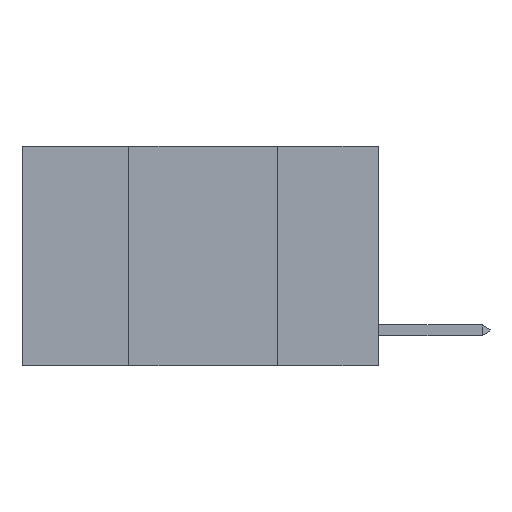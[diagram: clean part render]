
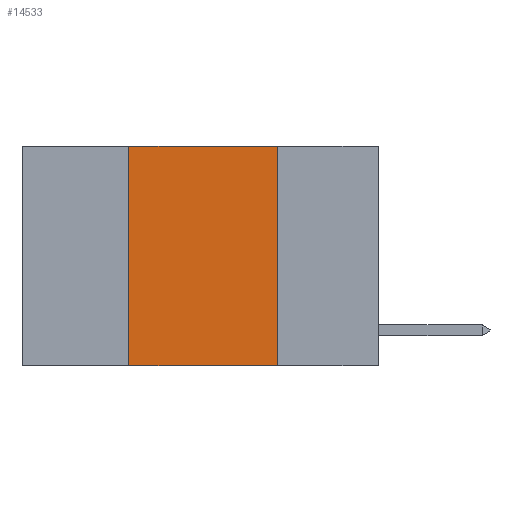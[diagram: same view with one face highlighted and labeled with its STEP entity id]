
A CAD part, left-side view. The second image highlights one B-rep face of the part: STEP entity #14533.
In plain terms, the highlighted planar face has unit normal (-1, 0, 0).
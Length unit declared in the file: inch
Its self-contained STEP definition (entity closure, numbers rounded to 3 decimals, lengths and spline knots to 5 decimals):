
#644 = LINE ( 'NONE', #12732, #9380 ) ;
#909 = AXIS2_PLACEMENT_3D ( 'NONE', #10828, #2904, #10870 ) ;
#1329 = CARTESIAN_POINT ( 'NONE',  ( 0., 0.6, 0. ) ) ;
#2159 = EDGE_LOOP ( 'NONE', ( #4464, #3932, #10152, #4290 ) ) ;
#2904 = DIRECTION ( 'NONE',  ( 1., 0., 0. ) ) ;
#3335 = EDGE_CURVE ( 'NONE', #10771, #10032, #644, .T. ) ;
#3684 = EDGE_CURVE ( 'NONE', #10666, #13697, #7776, .T. ) ;
#3932 = ORIENTED_EDGE ( 'NONE', *, *, #9842, .F. ) ;
#4290 = ORIENTED_EDGE ( 'NONE', *, *, #10112, .T. ) ;
#4464 = ORIENTED_EDGE ( 'NONE', *, *, #3684, .F. ) ;
#4695 = VECTOR ( 'NONE', #5255, 39.37008 ) ;
#5255 = DIRECTION ( 'NONE',  ( 0., -1., 0. ) ) ;
#7012 = DIRECTION ( 'NONE',  ( 0., 0., 1. ) ) ;
#7447 = CARTESIAN_POINT ( 'NONE',  ( 0., 0.6, -0.37 ) ) ;
#7700 = LINE ( 'NONE', #7447, #4695 ) ;
#7776 = LINE ( 'NONE', #13440, #10478 ) ;
#8603 = LINE ( 'NONE', #1329, #9301 ) ;
#9294 = DIRECTION ( 'NONE',  ( 0., -1., 0. ) ) ;
#9301 = VECTOR ( 'NONE', #9294, 39.37008 ) ;
#9380 = VECTOR ( 'NONE', #7012, 39.37008 ) ;
#9696 = PLANE ( 'NONE',  #909 ) ;
#9842 = EDGE_CURVE ( 'NONE', #10032, #10666, #8603, .T. ) ;
#9968 = DIRECTION ( 'NONE',  ( 0., 0., -1. ) ) ;
#10032 = VERTEX_POINT ( 'NONE', #13078 ) ;
#10112 = EDGE_CURVE ( 'NONE', #10771, #13697, #7700, .T. ) ;
#10152 = ORIENTED_EDGE ( 'NONE', *, *, #3335, .F. ) ;
#10478 = VECTOR ( 'NONE', #9968, 39.37008 ) ;
#10666 = VERTEX_POINT ( 'NONE', #14214 ) ;
#10771 = VERTEX_POINT ( 'NONE', #12170 ) ;
#10828 = CARTESIAN_POINT ( 'NONE',  ( 0., 0.6, 0. ) ) ;
#10870 = DIRECTION ( 'NONE',  ( 0., 0., -1. ) ) ;
#12170 = CARTESIAN_POINT ( 'NONE',  ( 0., 0.42, -0.37 ) ) ;
#12732 = CARTESIAN_POINT ( 'NONE',  ( 0., 0.42, 0. ) ) ;
#13078 = CARTESIAN_POINT ( 'NONE',  ( 0., 0.42, 0. ) ) ;
#13440 = CARTESIAN_POINT ( 'NONE',  ( 0., 0.17, 0. ) ) ;
#13697 = VERTEX_POINT ( 'NONE', #14011 ) ;
#13860 = FACE_OUTER_BOUND ( 'NONE', #2159, .T. ) ;
#14011 = CARTESIAN_POINT ( 'NONE',  ( 0., 0.17, -0.37 ) ) ;
#14214 = CARTESIAN_POINT ( 'NONE',  ( 0., 0.17, 0. ) ) ;
#14533 = ADVANCED_FACE ( 'NONE', ( #13860 ), #9696, .F. ) ;
